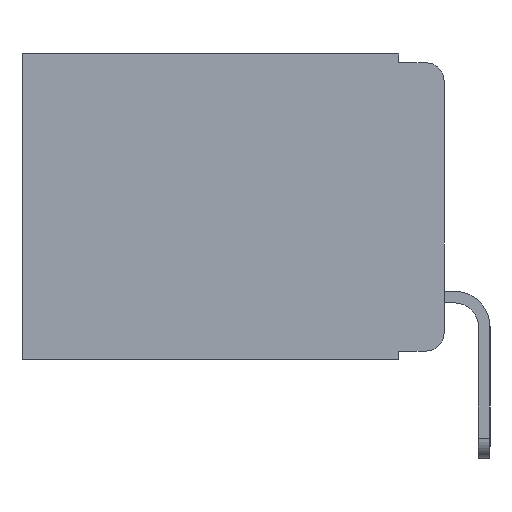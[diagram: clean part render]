
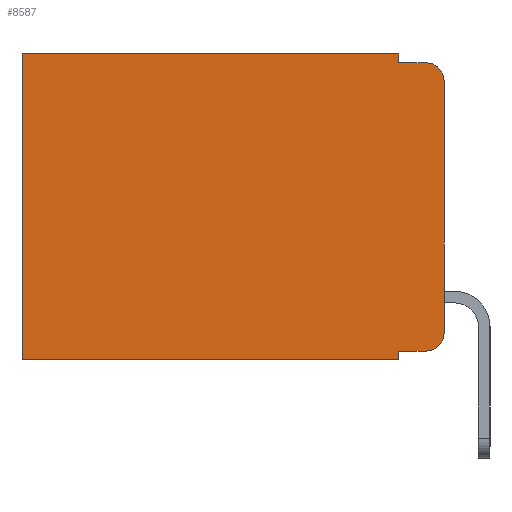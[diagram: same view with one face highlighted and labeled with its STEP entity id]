
A CAD part, left-side view. The second image highlights one B-rep face of the part: STEP entity #8587.
In plain terms, the highlighted planar face has unit normal (-1, 0, 0).
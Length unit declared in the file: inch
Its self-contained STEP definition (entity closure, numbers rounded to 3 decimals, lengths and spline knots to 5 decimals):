
#3 = DIRECTION ( 'NONE',  ( 0., 0., -1. ) ) ;
#221 = VERTEX_POINT ( 'NONE', #5377 ) ;
#238 = CARTESIAN_POINT ( 'NONE',  ( 0.298, 0.02, -0.333 ) ) ;
#324 = PLANE ( 'NONE',  #2985 ) ;
#393 = DIRECTION ( 'NONE',  ( 0., 1., 0. ) ) ;
#471 = VERTEX_POINT ( 'NONE', #4349 ) ;
#512 = VERTEX_POINT ( 'NONE', #238 ) ;
#542 = CARTESIAN_POINT ( 'NONE',  ( 0.298, 0.051, 0. ) ) ;
#865 = EDGE_CURVE ( 'NONE', #5020, #3624, #2455, .T. ) ;
#1194 = LINE ( 'NONE', #7193, #6861 ) ;
#1206 = VERTEX_POINT ( 'NONE', #542 ) ;
#1288 = LINE ( 'NONE', #10465, #9532 ) ;
#1897 = LINE ( 'NONE', #4208, #5452 ) ;
#2140 = VECTOR ( 'NONE', #7691, 39.37008 ) ;
#2455 = LINE ( 'NONE', #9135, #5872 ) ;
#2457 = AXIS2_PLACEMENT_3D ( 'NONE', #10377, #10634, #2766 ) ;
#2551 = VERTEX_POINT ( 'NONE', #7488 ) ;
#2766 = DIRECTION ( 'NONE',  ( 0., 0., -1. ) ) ;
#2768 = EDGE_CURVE ( 'NONE', #471, #3183, #1897, .T. ) ;
#2870 = CARTESIAN_POINT ( 'NONE',  ( 0.298, 0.02, -0.313 ) ) ;
#2985 = AXIS2_PLACEMENT_3D ( 'NONE', #7063, #10456, #3731 ) ;
#3049 = ORIENTED_EDGE ( 'NONE', *, *, #9323, .T. ) ;
#3102 = DIRECTION ( 'NONE',  ( 0., 0., -1. ) ) ;
#3183 = VERTEX_POINT ( 'NONE', #7647 ) ;
#3377 = VECTOR ( 'NONE', #7775, 39.37008 ) ;
#3479 = LINE ( 'NONE', #7577, #2140 ) ;
#3594 = ORIENTED_EDGE ( 'NONE', *, *, #7478, .F. ) ;
#3624 = VERTEX_POINT ( 'NONE', #7862 ) ;
#3650 = EDGE_CURVE ( 'NONE', #512, #5455, #10885, .T. ) ;
#3663 = CARTESIAN_POINT ( 'NONE',  ( 0.298, 0., -0.313 ) ) ;
#3731 = DIRECTION ( 'NONE',  ( 0., 0., -1. ) ) ;
#4208 = CARTESIAN_POINT ( 'NONE',  ( 0.298, 0.051, 0. ) ) ;
#4216 = EDGE_CURVE ( 'NONE', #3183, #3624, #9636, .T. ) ;
#4320 = VERTEX_POINT ( 'NONE', #7815 ) ;
#4349 = CARTESIAN_POINT ( 'NONE',  ( 0.298, 0.051, -0.333 ) ) ;
#4387 = CARTESIAN_POINT ( 'NONE',  ( 0.298, 0.473, 0. ) ) ;
#4415 = CARTESIAN_POINT ( 'NONE',  ( 0.298, 0., -0.343 ) ) ;
#4668 = EDGE_CURVE ( 'NONE', #471, #512, #8745, .T. ) ;
#5020 = VERTEX_POINT ( 'NONE', #4387 ) ;
#5264 = DIRECTION ( 'NONE',  ( 0., 0., -1. ) ) ;
#5377 = CARTESIAN_POINT ( 'NONE',  ( 0.298, 0., -0.03 ) ) ;
#5431 = ORIENTED_EDGE ( 'NONE', *, *, #865, .T. ) ;
#5452 = VECTOR ( 'NONE', #3, 39.37008 ) ;
#5455 = VERTEX_POINT ( 'NONE', #3663 ) ;
#5872 = VECTOR ( 'NONE', #9900, 39.37008 ) ;
#6308 = DIRECTION ( 'NONE',  ( -1., 0., 0. ) ) ;
#6861 = VECTOR ( 'NONE', #3102, 39.37008 ) ;
#6964 = DIRECTION ( 'NONE',  ( 0., -1., 0. ) ) ;
#7063 = CARTESIAN_POINT ( 'NONE',  ( 0.298, 0., 0. ) ) ;
#7193 = CARTESIAN_POINT ( 'NONE',  ( 0.298, 0., 0. ) ) ;
#7217 = VECTOR ( 'NONE', #8018, 39.37008 ) ;
#7478 = EDGE_CURVE ( 'NONE', #221, #5455, #1194, .T. ) ;
#7488 = CARTESIAN_POINT ( 'NONE',  ( 0.298, 0.02, -0.01 ) ) ;
#7577 = CARTESIAN_POINT ( 'NONE',  ( 0.298, 0.051, -0.01 ) ) ;
#7647 = CARTESIAN_POINT ( 'NONE',  ( 0.298, 0.051, -0.343 ) ) ;
#7691 = DIRECTION ( 'NONE',  ( 0., -1., 0. ) ) ;
#7775 = DIRECTION ( 'NONE',  ( 0., 0., -1. ) ) ;
#7815 = CARTESIAN_POINT ( 'NONE',  ( 0.298, 0.051, -0.01 ) ) ;
#7862 = CARTESIAN_POINT ( 'NONE',  ( 0.298, 0.473, -0.343 ) ) ;
#7900 = FACE_OUTER_BOUND ( 'NONE', #8163, .T. ) ;
#7956 = CARTESIAN_POINT ( 'NONE',  ( 0.298, 0.051, -0.333 ) ) ;
#8018 = DIRECTION ( 'NONE',  ( 0., 1., 0. ) ) ;
#8044 = ORIENTED_EDGE ( 'NONE', *, *, #10824, .F. ) ;
#8142 = ORIENTED_EDGE ( 'NONE', *, *, #8191, .T. ) ;
#8163 = EDGE_LOOP ( 'NONE', ( #3594, #3049, #8044, #8250, #8142, #5431, #8581, #10801, #10432, #10461 ) ) ;
#8191 = EDGE_CURVE ( 'NONE', #1206, #5020, #1288, .T. ) ;
#8250 = ORIENTED_EDGE ( 'NONE', *, *, #10001, .F. ) ;
#8581 = ORIENTED_EDGE ( 'NONE', *, *, #4216, .F. ) ;
#8587 = ADVANCED_FACE ( 'NONE', ( #7900 ), #324, .F. ) ;
#8745 = LINE ( 'NONE', #7956, #10247 ) ;
#8768 = AXIS2_PLACEMENT_3D ( 'NONE', #2870, #6308, #5264 ) ;
#9135 = CARTESIAN_POINT ( 'NONE',  ( 0.298, 0.473, 0. ) ) ;
#9323 = EDGE_CURVE ( 'NONE', #221, #2551, #10430, .T. ) ;
#9451 = CARTESIAN_POINT ( 'NONE',  ( 0.298, 0.051, 0. ) ) ;
#9532 = VECTOR ( 'NONE', #393, 39.37008 ) ;
#9636 = LINE ( 'NONE', #4415, #7217 ) ;
#9900 = DIRECTION ( 'NONE',  ( 0., 0., -1. ) ) ;
#10001 = EDGE_CURVE ( 'NONE', #1206, #4320, #10170, .T. ) ;
#10170 = LINE ( 'NONE', #9451, #3377 ) ;
#10247 = VECTOR ( 'NONE', #6964, 39.37008 ) ;
#10377 = CARTESIAN_POINT ( 'NONE',  ( 0.298, 0.02, -0.03 ) ) ;
#10430 = CIRCLE ( 'NONE', #2457, 0.02 ) ;
#10432 = ORIENTED_EDGE ( 'NONE', *, *, #4668, .T. ) ;
#10456 = DIRECTION ( 'NONE',  ( 1., 0., 0. ) ) ;
#10461 = ORIENTED_EDGE ( 'NONE', *, *, #3650, .T. ) ;
#10465 = CARTESIAN_POINT ( 'NONE',  ( 0.298, 0., 0. ) ) ;
#10634 = DIRECTION ( 'NONE',  ( -1., 0., 0. ) ) ;
#10801 = ORIENTED_EDGE ( 'NONE', *, *, #2768, .F. ) ;
#10824 = EDGE_CURVE ( 'NONE', #4320, #2551, #3479, .T. ) ;
#10885 = CIRCLE ( 'NONE', #8768, 0.02 ) ;
